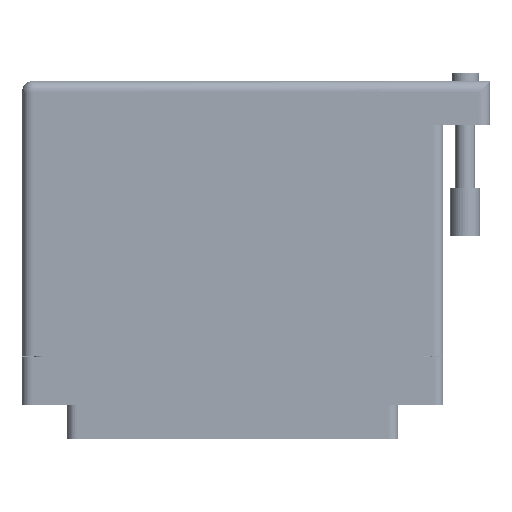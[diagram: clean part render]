
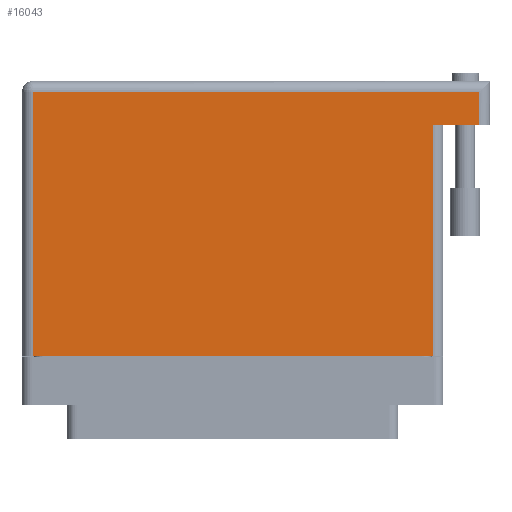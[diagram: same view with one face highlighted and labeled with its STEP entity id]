
A CAD part, front view. The second image highlights one B-rep face of the part: STEP entity #16043.
In plain terms, the highlighted face is planar.
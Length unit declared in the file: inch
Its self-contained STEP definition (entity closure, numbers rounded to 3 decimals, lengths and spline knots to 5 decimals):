
#1472 = CARTESIAN_POINT ( 'NONE',  ( -1.289, -0.1, 0.617 ) ) ;
#1494 = EDGE_CURVE ( 'NONE', #5785, #26828, #13789, .T. ) ;
#1649 = DIRECTION ( 'NONE',  ( 0., -1., 0. ) ) ;
#2726 = EDGE_LOOP ( 'NONE', ( #42383, #29075, #65191, #49865, #29004, #31179 ) ) ;
#3707 = EDGE_CURVE ( 'NONE', #21750, #40288, #46798, .T. ) ;
#4315 = AXIS2_PLACEMENT_3D ( 'NONE', #55994, #56711, #50751 ) ;
#5720 = LINE ( 'NONE', #13639, #16419 ) ;
#5785 = VERTEX_POINT ( 'NONE', #7181 ) ;
#6334 = VECTOR ( 'NONE', #1649, 39.37008 ) ;
#7181 = CARTESIAN_POINT ( 'NONE',  ( 1.589, 1.395, 0.617 ) ) ;
#7395 = DIRECTION ( 'NONE',  ( 0., 1., 0. ) ) ;
#11949 = CARTESIAN_POINT ( 'NONE',  ( 1.289, -0.1, 0.617 ) ) ;
#13639 = CARTESIAN_POINT ( 'NONE',  ( 1.589, 1.675, 0.617 ) ) ;
#13789 = LINE ( 'NONE', #24094, #27204 ) ;
#14814 = VECTOR ( 'NONE', #61406, 39.37008 ) ;
#16043 = ADVANCED_FACE ( 'NONE', ( #40843 ), #44559, .F. ) ;
#16419 = VECTOR ( 'NONE', #7395, 39.37008 ) ;
#19533 = VERTEX_POINT ( 'NONE', #33154 ) ;
#21341 = EDGE_CURVE ( 'NONE', #40288, #26828, #45503, .T. ) ;
#21750 = VERTEX_POINT ( 'NONE', #1472 ) ;
#24094 = CARTESIAN_POINT ( 'NONE',  ( 1.659, 1.395, 0.617 ) ) ;
#26828 = VERTEX_POINT ( 'NONE', #44088 ) ;
#27204 = VECTOR ( 'NONE', #70698, 39.37008 ) ;
#29004 = ORIENTED_EDGE ( 'NONE', *, *, #42315, .T. ) ;
#29075 = ORIENTED_EDGE ( 'NONE', *, *, #21341, .T. ) ;
#31179 = ORIENTED_EDGE ( 'NONE', *, *, #64708, .T. ) ;
#33154 = CARTESIAN_POINT ( 'NONE',  ( 1.589, 1.605, 0.617 ) ) ;
#34070 = EDGE_CURVE ( 'NONE', #5785, #19533, #5720, .T. ) ;
#36643 = LINE ( 'NONE', #47713, #6334 ) ;
#40288 = VERTEX_POINT ( 'NONE', #11949 ) ;
#40843 = FACE_OUTER_BOUND ( 'NONE', #2726, .T. ) ;
#42315 = EDGE_CURVE ( 'NONE', #19533, #53416, #73111, .T. ) ;
#42383 = ORIENTED_EDGE ( 'NONE', *, *, #3707, .T. ) ;
#43276 = CARTESIAN_POINT ( 'NONE',  ( -1.359, -0.1, 0.617 ) ) ;
#44088 = CARTESIAN_POINT ( 'NONE',  ( 1.289, 1.395, 0.617 ) ) ;
#44559 = PLANE ( 'NONE',  #4315 ) ;
#45503 = LINE ( 'NONE', #47601, #67733 ) ;
#46798 = LINE ( 'NONE', #43276, #14814 ) ;
#47601 = CARTESIAN_POINT ( 'NONE',  ( 1.289, 1.395, 0.617 ) ) ;
#47713 = CARTESIAN_POINT ( 'NONE',  ( -1.289, -0.1, 0.617 ) ) ;
#49865 = ORIENTED_EDGE ( 'NONE', *, *, #34070, .T. ) ;
#50751 = DIRECTION ( 'NONE',  ( -1., 0., 0. ) ) ;
#53416 = VERTEX_POINT ( 'NONE', #65758 ) ;
#54644 = DIRECTION ( 'NONE',  ( -1., 0., 0. ) ) ;
#55994 = CARTESIAN_POINT ( 'NONE',  ( -1.359, 1.675, 0.617 ) ) ;
#56711 = DIRECTION ( 'NONE',  ( 0., 0., -1. ) ) ;
#61406 = DIRECTION ( 'NONE',  ( 1., 0., 0. ) ) ;
#64708 = EDGE_CURVE ( 'NONE', #53416, #21750, #36643, .T. ) ;
#65191 = ORIENTED_EDGE ( 'NONE', *, *, #1494, .F. ) ;
#65264 = VECTOR ( 'NONE', #54644, 39.37008 ) ;
#65758 = CARTESIAN_POINT ( 'NONE',  ( -1.289, 1.605, 0.617 ) ) ;
#67733 = VECTOR ( 'NONE', #71893, 39.37008 ) ;
#70698 = DIRECTION ( 'NONE',  ( -1., 0., 0. ) ) ;
#71726 = CARTESIAN_POINT ( 'NONE',  ( -1.359, 1.605, 0.617 ) ) ;
#71893 = DIRECTION ( 'NONE',  ( 0., 1., 0. ) ) ;
#73111 = LINE ( 'NONE', #71726, #65264 ) ;
